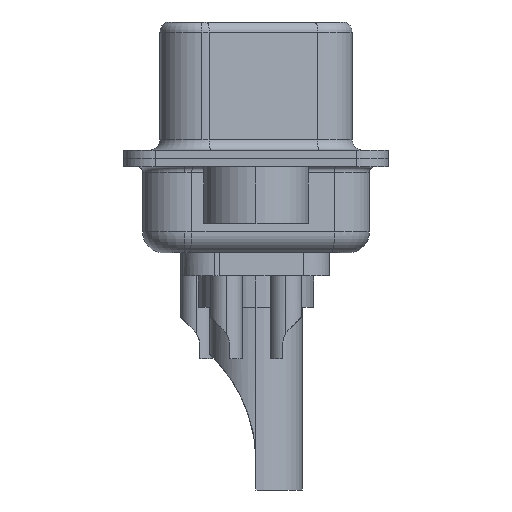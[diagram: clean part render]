
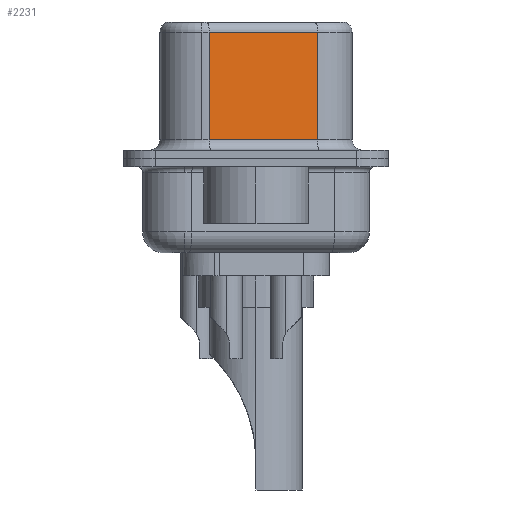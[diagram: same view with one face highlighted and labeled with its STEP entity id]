
A CAD part, left-side view. The second image highlights one B-rep face of the part: STEP entity #2231.
In plain terms, the highlighted planar face has unit normal (-0.985, -0.174, 0).
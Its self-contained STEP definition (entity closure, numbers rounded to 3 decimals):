
#599 = EDGE_CURVE ( 'NONE', #959, #18839, #2570, .T. ) ;
#959 = VERTEX_POINT ( 'NONE', #12005 ) ;
#1390 = EDGE_CURVE ( 'NONE', #959, #15685, #17291, .T. ) ;
#2231 = ADVANCED_FACE ( 'NONE', ( #6609 ), #6789, .F. ) ;
#2570 = LINE ( 'NONE', #16243, #9383 ) ;
#4265 = CARTESIAN_POINT ( 'NONE',  ( 3.675, 2.233, 6.52 ) ) ;
#4292 = VERTEX_POINT ( 'NONE', #9461 ) ;
#5167 = EDGE_CURVE ( 'NONE', #4292, #15685, #12569, .T. ) ;
#5449 = CARTESIAN_POINT ( 'NONE',  ( 3.675, 2.233, 6.02 ) ) ;
#5584 = ORIENTED_EDGE ( 'NONE', *, *, #5167, .T. ) ;
#6461 = CARTESIAN_POINT ( 'NONE',  ( 4.585, -2.927, 0.9 ) ) ;
#6609 = FACE_OUTER_BOUND ( 'NONE', #13411, .T. ) ;
#6789 = PLANE ( 'NONE',  #15547 ) ;
#8409 = DIRECTION ( 'NONE',  ( -0.174, 0.985, 0. ) ) ;
#8552 = DIRECTION ( 'NONE',  ( 0.985, 0.174, 0. ) ) ;
#9383 = VECTOR ( 'NONE', #17975, 1000. ) ;
#9384 = ORIENTED_EDGE ( 'NONE', *, *, #19353, .T. ) ;
#9461 = CARTESIAN_POINT ( 'NONE',  ( 3.675, 2.233, 0.9 ) ) ;
#11249 = CARTESIAN_POINT ( 'NONE',  ( 4.585, -2.927, 6.52 ) ) ;
#11486 = VECTOR ( 'NONE', #18618, 1000. ) ;
#11607 = CARTESIAN_POINT ( 'NONE',  ( 4.585, -2.927, 0.9 ) ) ;
#12005 = CARTESIAN_POINT ( 'NONE',  ( 4.585, -2.927, 6.02 ) ) ;
#12265 = ORIENTED_EDGE ( 'NONE', *, *, #1390, .F. ) ;
#12569 = LINE ( 'NONE', #6461, #19905 ) ;
#13357 = CARTESIAN_POINT ( 'NONE',  ( 4.585, -2.927, 6.52 ) ) ;
#13411 = EDGE_LOOP ( 'NONE', ( #12265, #20672, #9384, #5584 ) ) ;
#14722 = VECTOR ( 'NONE', #20449, 1000. ) ;
#15547 = AXIS2_PLACEMENT_3D ( 'NONE', #13357, #8552, #8409 ) ;
#15685 = VERTEX_POINT ( 'NONE', #11607 ) ;
#16243 = CARTESIAN_POINT ( 'NONE',  ( 4.585, -2.927, 6.02 ) ) ;
#16585 = DIRECTION ( 'NONE',  ( 0.174, -0.985, 0. ) ) ;
#17291 = LINE ( 'NONE', #11249, #14722 ) ;
#17975 = DIRECTION ( 'NONE',  ( -0.174, 0.985, 0. ) ) ;
#18618 = DIRECTION ( 'NONE',  ( 0., 0., -1. ) ) ;
#18839 = VERTEX_POINT ( 'NONE', #5449 ) ;
#19353 = EDGE_CURVE ( 'NONE', #18839, #4292, #20124, .T. ) ;
#19905 = VECTOR ( 'NONE', #16585, 1000. ) ;
#20124 = LINE ( 'NONE', #4265, #11486 ) ;
#20449 = DIRECTION ( 'NONE',  ( 0., 0., -1. ) ) ;
#20672 = ORIENTED_EDGE ( 'NONE', *, *, #599, .T. ) ;
